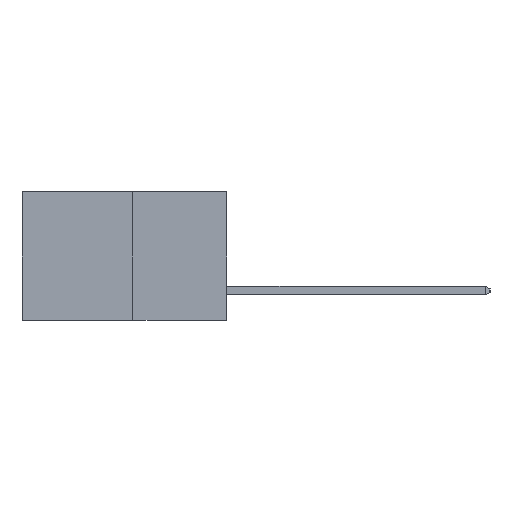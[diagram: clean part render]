
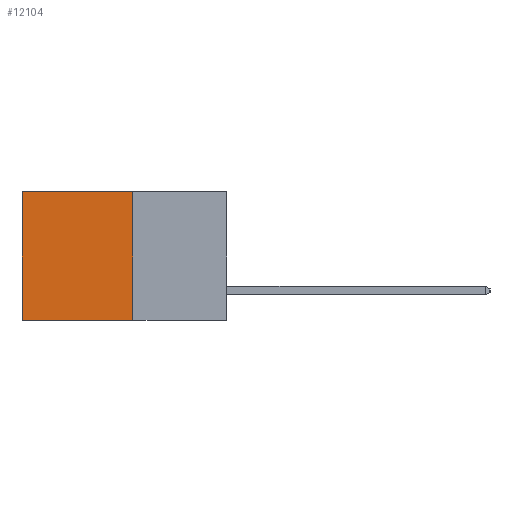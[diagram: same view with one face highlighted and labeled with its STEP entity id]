
A CAD part, left-side view. The second image highlights one B-rep face of the part: STEP entity #12104.
In plain terms, the highlighted planar face has unit normal (-1, 0, 0).
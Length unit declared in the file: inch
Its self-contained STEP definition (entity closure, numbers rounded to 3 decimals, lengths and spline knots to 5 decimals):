
#352 = EDGE_LOOP ( 'NONE', ( #10828, #8649, #2008, #7334 ) ) ;
#615 = LINE ( 'NONE', #995, #2845 ) ;
#995 = CARTESIAN_POINT ( 'NONE',  ( 0.277, 0.27, -0.37 ) ) ;
#2008 = ORIENTED_EDGE ( 'NONE', *, *, #3754, .F. ) ;
#2185 = CARTESIAN_POINT ( 'NONE',  ( 0.277, 0.59, 0. ) ) ;
#2331 = DIRECTION ( 'NONE',  ( 0., 0., -1. ) ) ;
#2370 = LINE ( 'NONE', #5570, #9564 ) ;
#2501 = LINE ( 'NONE', #7144, #12106 ) ;
#2824 = VECTOR ( 'NONE', #5073, 39.37008 ) ;
#2845 = VECTOR ( 'NONE', #4797, 39.37008 ) ;
#3350 = CARTESIAN_POINT ( 'NONE',  ( 0.277, 0.27, -0.37 ) ) ;
#3537 = VERTEX_POINT ( 'NONE', #8375 ) ;
#3754 = EDGE_CURVE ( 'NONE', #3537, #4820, #9721, .T. ) ;
#3972 = EDGE_CURVE ( 'NONE', #8826, #10318, #2370, .T. ) ;
#4089 = PLANE ( 'NONE',  #11317 ) ;
#4557 = EDGE_CURVE ( 'NONE', #3537, #8826, #2501, .T. ) ;
#4797 = DIRECTION ( 'NONE',  ( 0., 1., 0. ) ) ;
#4820 = VERTEX_POINT ( 'NONE', #3350 ) ;
#4999 = DIRECTION ( 'NONE',  ( 1., 0., 0. ) ) ;
#5073 = DIRECTION ( 'NONE',  ( 0., 0., -1. ) ) ;
#5570 = CARTESIAN_POINT ( 'NONE',  ( 0.277, 0.59, -0.37 ) ) ;
#6521 = EDGE_CURVE ( 'NONE', #4820, #10318, #615, .T. ) ;
#7144 = CARTESIAN_POINT ( 'NONE',  ( 0.277, 0.27, 0. ) ) ;
#7169 = DIRECTION ( 'NONE',  ( 0., 1., 0. ) ) ;
#7334 = ORIENTED_EDGE ( 'NONE', *, *, #4557, .T. ) ;
#8327 = CARTESIAN_POINT ( 'NONE',  ( 0.277, 0.27, -0.37 ) ) ;
#8375 = CARTESIAN_POINT ( 'NONE',  ( 0.277, 0.27, 0. ) ) ;
#8649 = ORIENTED_EDGE ( 'NONE', *, *, #6521, .F. ) ;
#8826 = VERTEX_POINT ( 'NONE', #2185 ) ;
#9564 = VECTOR ( 'NONE', #2331, 39.37008 ) ;
#9721 = LINE ( 'NONE', #8327, #2824 ) ;
#10239 = CARTESIAN_POINT ( 'NONE',  ( 0.277, 0.59, -0.37 ) ) ;
#10318 = VERTEX_POINT ( 'NONE', #10239 ) ;
#10609 = FACE_OUTER_BOUND ( 'NONE', #352, .T. ) ;
#10636 = CARTESIAN_POINT ( 'NONE',  ( 0.277, 0.27, -0.37 ) ) ;
#10828 = ORIENTED_EDGE ( 'NONE', *, *, #3972, .T. ) ;
#11317 = AXIS2_PLACEMENT_3D ( 'NONE', #10636, #4999, #11519 ) ;
#11519 = DIRECTION ( 'NONE',  ( 0., 0., -1. ) ) ;
#12104 = ADVANCED_FACE ( 'NONE', ( #10609 ), #4089, .F. ) ;
#12106 = VECTOR ( 'NONE', #7169, 39.37008 ) ;
